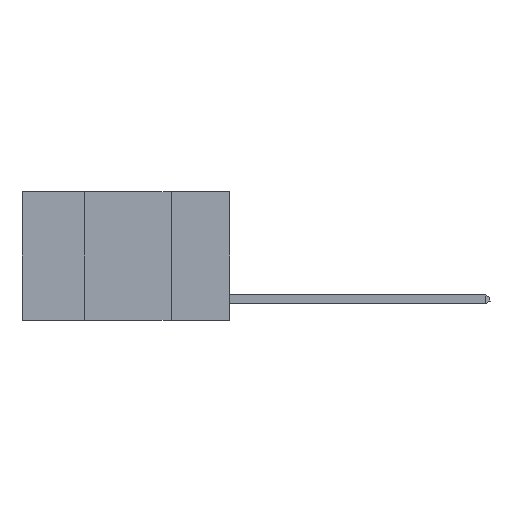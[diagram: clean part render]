
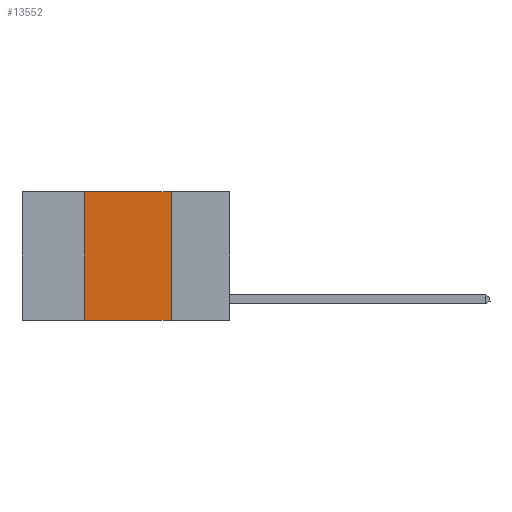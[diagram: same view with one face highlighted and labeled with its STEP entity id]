
A CAD part, left-side view. The second image highlights one B-rep face of the part: STEP entity #13552.
In plain terms, the highlighted planar face has unit normal (-1, 0, 0).
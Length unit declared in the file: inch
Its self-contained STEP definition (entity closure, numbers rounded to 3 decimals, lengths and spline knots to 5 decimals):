
#355 = DIRECTION ( 'NONE',  ( 0., 0., -1. ) ) ;
#468 = AXIS2_PLACEMENT_3D ( 'NONE', #14932, #7671, #355 ) ;
#685 = EDGE_CURVE ( 'NONE', #13026, #1460, #9030, .T. ) ;
#1111 = FACE_OUTER_BOUND ( 'NONE', #4008, .T. ) ;
#1319 = ORIENTED_EDGE ( 'NONE', *, *, #685, .F. ) ;
#1460 = VERTEX_POINT ( 'NONE', #13163 ) ;
#1468 = VECTOR ( 'NONE', #15016, 39.37008 ) ;
#2178 = CARTESIAN_POINT ( 'NONE',  ( 0., 0.17, -0.37 ) ) ;
#2333 = EDGE_CURVE ( 'NONE', #11833, #13241, #14399, .T. ) ;
#2489 = VECTOR ( 'NONE', #6695, 39.37008 ) ;
#2880 = CARTESIAN_POINT ( 'NONE',  ( 0., 0.17, 0. ) ) ;
#4008 = EDGE_LOOP ( 'NONE', ( #10489, #8572, #1319, #13554 ) ) ;
#4544 = DIRECTION ( 'NONE',  ( 0., -1., 0. ) ) ;
#4566 = CARTESIAN_POINT ( 'NONE',  ( 0., 0.6, -0.37 ) ) ;
#5322 = CARTESIAN_POINT ( 'NONE',  ( 0., 0.17, 0. ) ) ;
#6695 = DIRECTION ( 'NONE',  ( 0., 0., 1. ) ) ;
#6971 = DIRECTION ( 'NONE',  ( 0., -1., 0. ) ) ;
#7671 = DIRECTION ( 'NONE',  ( 1., 0., 0. ) ) ;
#8572 = ORIENTED_EDGE ( 'NONE', *, *, #11420, .F. ) ;
#9030 = LINE ( 'NONE', #12331, #2489 ) ;
#9281 = VECTOR ( 'NONE', #6971, 39.37008 ) ;
#9773 = LINE ( 'NONE', #14247, #13359 ) ;
#10489 = ORIENTED_EDGE ( 'NONE', *, *, #2333, .F. ) ;
#11270 = PLANE ( 'NONE',  #468 ) ;
#11420 = EDGE_CURVE ( 'NONE', #1460, #11833, #9773, .T. ) ;
#11833 = VERTEX_POINT ( 'NONE', #2880 ) ;
#12331 = CARTESIAN_POINT ( 'NONE',  ( 0., 0.42, 0. ) ) ;
#12404 = CARTESIAN_POINT ( 'NONE',  ( 0., 0.42, -0.37 ) ) ;
#13026 = VERTEX_POINT ( 'NONE', #12404 ) ;
#13163 = CARTESIAN_POINT ( 'NONE',  ( 0., 0.42, 0. ) ) ;
#13241 = VERTEX_POINT ( 'NONE', #2178 ) ;
#13359 = VECTOR ( 'NONE', #4544, 39.37008 ) ;
#13552 = ADVANCED_FACE ( 'NONE', ( #1111 ), #11270, .F. ) ;
#13554 = ORIENTED_EDGE ( 'NONE', *, *, #15653, .T. ) ;
#14247 = CARTESIAN_POINT ( 'NONE',  ( 0., 0.6, 0. ) ) ;
#14399 = LINE ( 'NONE', #5322, #1468 ) ;
#14932 = CARTESIAN_POINT ( 'NONE',  ( 0., 0.6, 0. ) ) ;
#15016 = DIRECTION ( 'NONE',  ( 0., 0., -1. ) ) ;
#15653 = EDGE_CURVE ( 'NONE', #13026, #13241, #15710, .T. ) ;
#15710 = LINE ( 'NONE', #4566, #9281 ) ;
